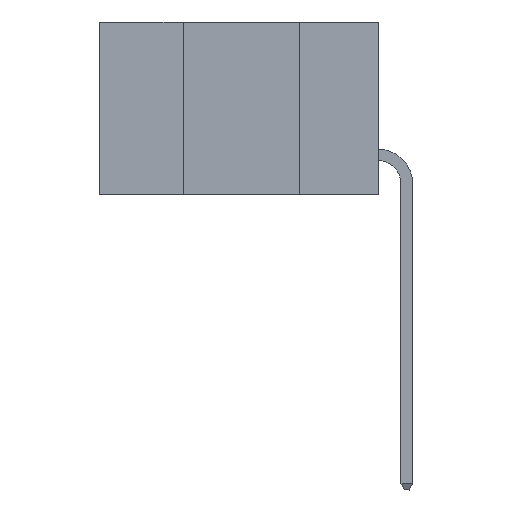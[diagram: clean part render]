
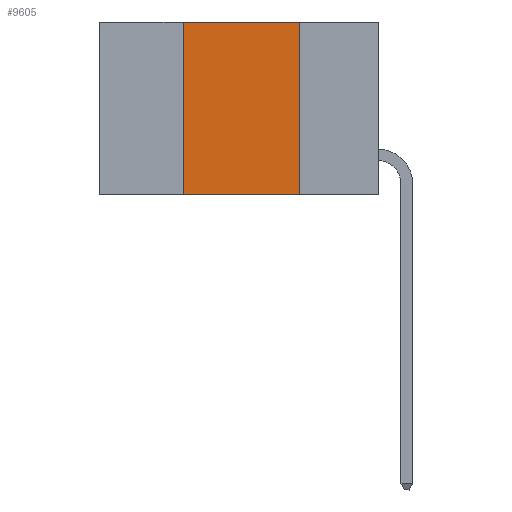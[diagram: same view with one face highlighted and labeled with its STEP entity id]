
A CAD part, left-side view. The second image highlights one B-rep face of the part: STEP entity #9605.
In plain terms, the highlighted planar face has unit normal (-1, 0, 0).
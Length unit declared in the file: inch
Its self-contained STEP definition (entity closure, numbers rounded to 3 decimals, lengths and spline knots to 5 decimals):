
#96 = DIRECTION ( 'NONE',  ( 0., 0., 1. ) ) ;
#479 = ORIENTED_EDGE ( 'NONE', *, *, #6032, .T. ) ;
#1618 = ORIENTED_EDGE ( 'NONE', *, *, #2446, .F. ) ;
#1691 = DIRECTION ( 'NONE',  ( 0., -1., 0. ) ) ;
#2446 = EDGE_CURVE ( 'NONE', #9744, #7947, #5382, .T. ) ;
#2484 = CARTESIAN_POINT ( 'NONE',  ( 0., 0.17, -0.37 ) ) ;
#2734 = LINE ( 'NONE', #8748, #5328 ) ;
#4219 = PLANE ( 'NONE',  #12004 ) ;
#5328 = VECTOR ( 'NONE', #1691, 39.37008 ) ;
#5382 = LINE ( 'NONE', #2484, #11916 ) ;
#5436 = VERTEX_POINT ( 'NONE', #9471 ) ;
#6032 = EDGE_CURVE ( 'NONE', #5436, #7947, #6287, .T. ) ;
#6287 = LINE ( 'NONE', #10580, #9137 ) ;
#7018 = EDGE_LOOP ( 'NONE', ( #1618, #7465, #8854, #479 ) ) ;
#7125 = LINE ( 'NONE', #11046, #8243 ) ;
#7241 = CARTESIAN_POINT ( 'NONE',  ( 0., 0.42, 0. ) ) ;
#7300 = DIRECTION ( 'NONE',  ( 1., 0., 0. ) ) ;
#7344 = VERTEX_POINT ( 'NONE', #7241 ) ;
#7465 = ORIENTED_EDGE ( 'NONE', *, *, #9041, .F. ) ;
#7497 = CARTESIAN_POINT ( 'NONE',  ( 0., 0.17, 0. ) ) ;
#7553 = CARTESIAN_POINT ( 'NONE',  ( 0., 0.17, -0.37 ) ) ;
#7947 = VERTEX_POINT ( 'NONE', #7553 ) ;
#8243 = VECTOR ( 'NONE', #96, 39.37008 ) ;
#8475 = EDGE_CURVE ( 'NONE', #5436, #7344, #7125, .T. ) ;
#8595 = DIRECTION ( 'NONE',  ( 0., -1., 0. ) ) ;
#8748 = CARTESIAN_POINT ( 'NONE',  ( 0., 0.6, 0. ) ) ;
#8854 = ORIENTED_EDGE ( 'NONE', *, *, #8475, .F. ) ;
#9041 = EDGE_CURVE ( 'NONE', #7344, #9744, #2734, .T. ) ;
#9137 = VECTOR ( 'NONE', #8595, 39.37008 ) ;
#9471 = CARTESIAN_POINT ( 'NONE',  ( 0., 0.42, -0.37 ) ) ;
#9605 = ADVANCED_FACE ( 'NONE', ( #10082 ), #4219, .F. ) ;
#9744 = VERTEX_POINT ( 'NONE', #7497 ) ;
#10082 = FACE_OUTER_BOUND ( 'NONE', #7018, .T. ) ;
#10580 = CARTESIAN_POINT ( 'NONE',  ( 0., 0.6, -0.37 ) ) ;
#11046 = CARTESIAN_POINT ( 'NONE',  ( 0., 0.42, -0.37 ) ) ;
#11332 = CARTESIAN_POINT ( 'NONE',  ( 0., 0.6, 0. ) ) ;
#11916 = VECTOR ( 'NONE', #12213, 39.37008 ) ;
#12004 = AXIS2_PLACEMENT_3D ( 'NONE', #11332, #7300, #12335 ) ;
#12213 = DIRECTION ( 'NONE',  ( 0., 0., -1. ) ) ;
#12335 = DIRECTION ( 'NONE',  ( 0., 0., -1. ) ) ;
